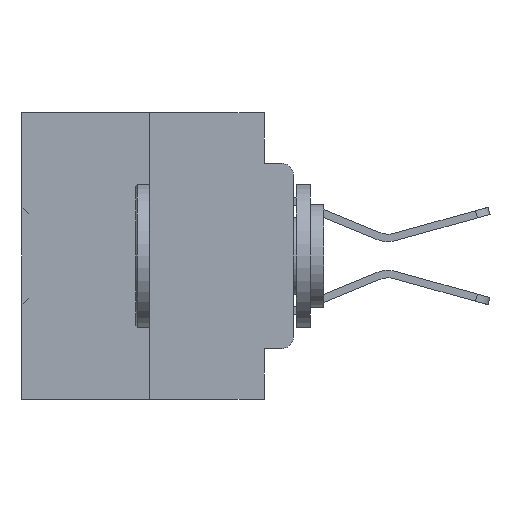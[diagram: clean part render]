
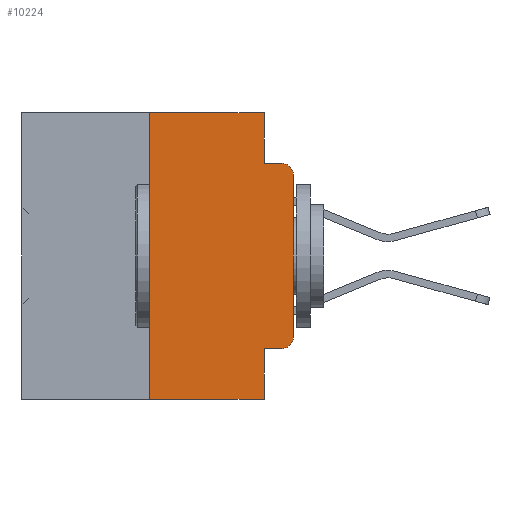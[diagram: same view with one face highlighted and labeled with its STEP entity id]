
A CAD part, left-side view. The second image highlights one B-rep face of the part: STEP entity #10224.
In plain terms, the highlighted planar face has unit normal (-1, 0, 0).
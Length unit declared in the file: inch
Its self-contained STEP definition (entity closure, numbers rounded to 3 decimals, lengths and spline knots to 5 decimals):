
#160 = CARTESIAN_POINT ( 'NONE',  ( 0., 0.02, -0.4115 ) ) ;
#497 = CARTESIAN_POINT ( 'NONE',  ( 0., 0.02, -0.1085 ) ) ;
#590 = PLANE ( 'NONE',  #21793 ) ;
#972 = EDGE_CURVE ( 'NONE', #23622, #31617, #31559, .T. ) ;
#1147 = VERTEX_POINT ( 'NONE', #11467 ) ;
#1588 = VERTEX_POINT ( 'NONE', #7577 ) ;
#1704 = CARTESIAN_POINT ( 'NONE',  ( 0., 0.02, -0.0885 ) ) ;
#1749 = DIRECTION ( 'NONE',  ( 0., 0., -1. ) ) ;
#2687 = ORIENTED_EDGE ( 'NONE', *, *, #20835, .T. ) ;
#2954 = CARTESIAN_POINT ( 'NONE',  ( 0., 0.25, 0. ) ) ;
#3259 = EDGE_LOOP ( 'NONE', ( #10293, #2687, #6612, #19956, #39089, #3447, #27753, #21991, #24336, #14030 ) ) ;
#3447 = ORIENTED_EDGE ( 'NONE', *, *, #22499, .F. ) ;
#4622 = LINE ( 'NONE', #10500, #25394 ) ;
#4710 = EDGE_CURVE ( 'NONE', #37727, #23622, #4925, .T. ) ;
#4925 = CIRCLE ( 'NONE', #10098, 0.02 ) ;
#5206 = CARTESIAN_POINT ( 'NONE',  ( 0., 0.051, -0.5 ) ) ;
#5638 = DIRECTION ( 'NONE',  ( 0., -1., 0. ) ) ;
#5994 = DIRECTION ( 'NONE',  ( 0., 0., -1. ) ) ;
#6458 = FACE_OUTER_BOUND ( 'NONE', #3259, .T. ) ;
#6612 = ORIENTED_EDGE ( 'NONE', *, *, #25692, .F. ) ;
#7065 = DIRECTION ( 'NONE',  ( 0., -1., 0. ) ) ;
#7239 = VECTOR ( 'NONE', #30197, 39.37008 ) ;
#7577 = CARTESIAN_POINT ( 'NONE',  ( 0., 0.051, -0.0885 ) ) ;
#8592 = VECTOR ( 'NONE', #1749, 39.37008 ) ;
#9043 = DIRECTION ( 'NONE',  ( -1., 0., 0. ) ) ;
#9085 = VERTEX_POINT ( 'NONE', #5206 ) ;
#10098 = AXIS2_PLACEMENT_3D ( 'NONE', #24412, #9043, #5994 ) ;
#10186 = DIRECTION ( 'NONE',  ( 0., -1., 0. ) ) ;
#10224 = ADVANCED_FACE ( 'NONE', ( #6458 ), #590, .F. ) ;
#10293 = ORIENTED_EDGE ( 'NONE', *, *, #972, .T. ) ;
#10500 = CARTESIAN_POINT ( 'NONE',  ( 0., 0.473, -0.5 ) ) ;
#11357 = CARTESIAN_POINT ( 'NONE',  ( 0., 0.25, 0. ) ) ;
#11454 = CARTESIAN_POINT ( 'NONE',  ( 0., 0.051, -0.4115 ) ) ;
#11467 = CARTESIAN_POINT ( 'NONE',  ( 0., 0.051, 0. ) ) ;
#12669 = VECTOR ( 'NONE', #23287, 39.37008 ) ;
#12735 = DIRECTION ( 'NONE',  ( 1., 0., 0. ) ) ;
#12848 = DIRECTION ( 'NONE',  ( -1., 0., 0. ) ) ;
#13295 = CARTESIAN_POINT ( 'NONE',  ( 0., 0., 0. ) ) ;
#14030 = ORIENTED_EDGE ( 'NONE', *, *, #4710, .T. ) ;
#14608 = VERTEX_POINT ( 'NONE', #11454 ) ;
#14698 = CARTESIAN_POINT ( 'NONE',  ( 0., 0.051, 0. ) ) ;
#15548 = EDGE_CURVE ( 'NONE', #14608, #37727, #38784, .T. ) ;
#16364 = CARTESIAN_POINT ( 'NONE',  ( 0., 0.051, -0.0885 ) ) ;
#17226 = CARTESIAN_POINT ( 'NONE',  ( 0., 0.051, -0.4115 ) ) ;
#18222 = CARTESIAN_POINT ( 'NONE',  ( 0., 0.25, -0.5 ) ) ;
#19956 = ORIENTED_EDGE ( 'NONE', *, *, #32715, .F. ) ;
#20348 = LINE ( 'NONE', #14698, #8592 ) ;
#20835 = EDGE_CURVE ( 'NONE', #31617, #29079, #33037, .T. ) ;
#21345 = VECTOR ( 'NONE', #22265, 39.37008 ) ;
#21793 = AXIS2_PLACEMENT_3D ( 'NONE', #37691, #12735, #27742 ) ;
#21991 = ORIENTED_EDGE ( 'NONE', *, *, #23308, .F. ) ;
#22265 = DIRECTION ( 'NONE',  ( 0., 0., -1. ) ) ;
#22496 = VERTEX_POINT ( 'NONE', #18222 ) ;
#22499 = EDGE_CURVE ( 'NONE', #22496, #23449, #39160, .T. ) ;
#22742 = CARTESIAN_POINT ( 'NONE',  ( 0., 0., -0.3915 ) ) ;
#23287 = DIRECTION ( 'NONE',  ( 0., -1., 0. ) ) ;
#23308 = EDGE_CURVE ( 'NONE', #14608, #9085, #20348, .T. ) ;
#23449 = VERTEX_POINT ( 'NONE', #2954 ) ;
#23622 = VERTEX_POINT ( 'NONE', #22742 ) ;
#23667 = CARTESIAN_POINT ( 'NONE',  ( 0., 0., -0.1085 ) ) ;
#24336 = ORIENTED_EDGE ( 'NONE', *, *, #15548, .T. ) ;
#24412 = CARTESIAN_POINT ( 'NONE',  ( 0., 0.02, -0.3915 ) ) ;
#25179 = DIRECTION ( 'NONE',  ( 0., 0., -1. ) ) ;
#25394 = VECTOR ( 'NONE', #7065, 39.37008 ) ;
#25507 = LINE ( 'NONE', #29177, #21345 ) ;
#25692 = EDGE_CURVE ( 'NONE', #1588, #29079, #37270, .T. ) ;
#27742 = DIRECTION ( 'NONE',  ( 0., 0., -1. ) ) ;
#27753 = ORIENTED_EDGE ( 'NONE', *, *, #36006, .T. ) ;
#29033 = CARTESIAN_POINT ( 'NONE',  ( 0., 0.473, 0. ) ) ;
#29079 = VERTEX_POINT ( 'NONE', #1704 ) ;
#29177 = CARTESIAN_POINT ( 'NONE',  ( 0., 0.051, 0. ) ) ;
#29626 = VECTOR ( 'NONE', #10186, 39.37008 ) ;
#29777 = EDGE_CURVE ( 'NONE', #23449, #1147, #32070, .T. ) ;
#30197 = DIRECTION ( 'NONE',  ( 0., 0., 1. ) ) ;
#31559 = LINE ( 'NONE', #13295, #32819 ) ;
#31617 = VERTEX_POINT ( 'NONE', #23667 ) ;
#32070 = LINE ( 'NONE', #29033, #29626 ) ;
#32715 = EDGE_CURVE ( 'NONE', #1147, #1588, #25507, .T. ) ;
#32819 = VECTOR ( 'NONE', #34409, 39.37008 ) ;
#33037 = CIRCLE ( 'NONE', #35653, 0.02 ) ;
#34409 = DIRECTION ( 'NONE',  ( 0., 0., 1. ) ) ;
#35331 = VECTOR ( 'NONE', #5638, 39.37008 ) ;
#35653 = AXIS2_PLACEMENT_3D ( 'NONE', #497, #12848, #25179 ) ;
#36006 = EDGE_CURVE ( 'NONE', #22496, #9085, #4622, .T. ) ;
#37270 = LINE ( 'NONE', #16364, #35331 ) ;
#37691 = CARTESIAN_POINT ( 'NONE',  ( 0., 0.473, 0. ) ) ;
#37727 = VERTEX_POINT ( 'NONE', #160 ) ;
#38784 = LINE ( 'NONE', #17226, #12669 ) ;
#39089 = ORIENTED_EDGE ( 'NONE', *, *, #29777, .F. ) ;
#39160 = LINE ( 'NONE', #11357, #7239 ) ;
